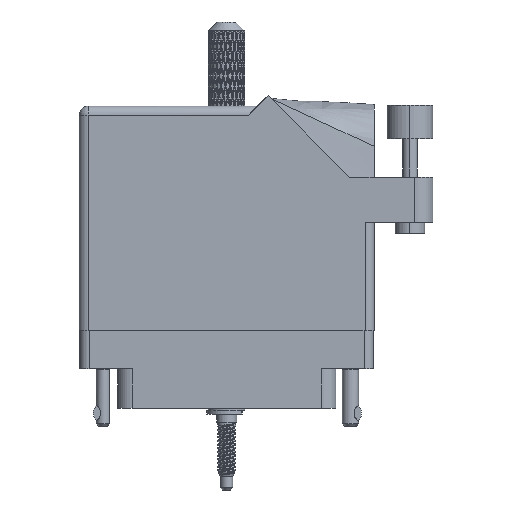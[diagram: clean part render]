
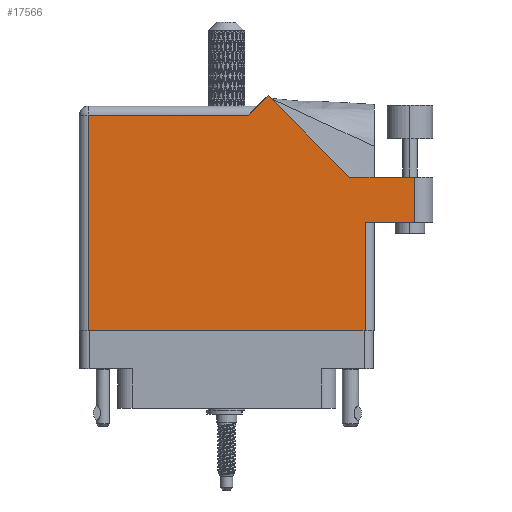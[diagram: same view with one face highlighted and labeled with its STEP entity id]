
A CAD part, front view. The second image highlights one B-rep face of the part: STEP entity #17566.
In plain terms, the highlighted face is planar.
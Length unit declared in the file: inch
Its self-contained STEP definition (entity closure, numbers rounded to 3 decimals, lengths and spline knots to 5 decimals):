
#2791 = DIRECTION ( 'NONE',  ( -0.707, -0.707, 0. ) ) ;
#10307 = LINE ( 'NONE', #37075, #46090 ) ;
#12872 = VERTEX_POINT ( 'NONE', #85176 ) ;
#12920 = DIRECTION ( 'NONE',  ( -1., 0., 0. ) ) ;
#13044 = DIRECTION ( 'NONE',  ( 1., 0., 0. ) ) ;
#15157 = CARTESIAN_POINT ( 'NONE',  ( 1.948, 0.737, 0. ) ) ;
#16138 = AXIS2_PLACEMENT_3D ( 'NONE', #21822, #30300, #65587 ) ;
#16716 = VERTEX_POINT ( 'NONE', #63586 ) ;
#17566 = ADVANCED_FACE ( 'NONE', ( #80615 ), #40283, .F. ) ;
#18502 = DIRECTION ( 'NONE',  ( 0., 1., 0. ) ) ;
#21059 = LINE ( 'NONE', #15157, #89837 ) ;
#21822 = CARTESIAN_POINT ( 'NONE',  ( 0., 1.53, 0. ) ) ;
#22752 = EDGE_LOOP ( 'NONE', ( #46769, #24610, #47847, #94055, #78422, #37450, #82139, #95733, #101850 ) ) ;
#24610 = ORIENTED_EDGE ( 'NONE', *, *, #84553, .T. ) ;
#25171 = EDGE_CURVE ( 'NONE', #108769, #67996, #77918, .T. ) ;
#26047 = CARTESIAN_POINT ( 'NONE',  ( 0., 0., 0. ) ) ;
#26942 = DIRECTION ( 'NONE',  ( -0.707, 0.707, 0. ) ) ;
#28655 = VERTEX_POINT ( 'NONE', #44791 ) ;
#30300 = DIRECTION ( 'NONE',  ( 0., 0., -1. ) ) ;
#32064 = VECTOR ( 'NONE', #40849, 39.37008 ) ;
#32855 = EDGE_CURVE ( 'NONE', #108062, #96433, #21059, .T. ) ;
#32898 = CARTESIAN_POINT ( 'NONE',  ( 1.948, 0., 0. ) ) ;
#34524 = VECTOR ( 'NONE', #43389, 39.37008 ) ;
#34803 = EDGE_CURVE ( 'NONE', #12872, #108062, #49649, .T. ) ;
#35279 = LINE ( 'NONE', #109047, #110829 ) ;
#37075 = CARTESIAN_POINT ( 'NONE',  ( 1.217, 1.53, 0. ) ) ;
#37450 = ORIENTED_EDGE ( 'NONE', *, *, #52442, .T. ) ;
#39596 = CARTESIAN_POINT ( 'NONE',  ( 0.062, 1.468, 0. ) ) ;
#40283 = PLANE ( 'NONE',  #16138 ) ;
#40849 = DIRECTION ( 'NONE',  ( -1., 0., 0. ) ) ;
#41670 = CARTESIAN_POINT ( 'NONE',  ( 0.062, 0., 0. ) ) ;
#43389 = DIRECTION ( 'NONE',  ( 1., 0., 0. ) ) ;
#44791 = CARTESIAN_POINT ( 'NONE',  ( 1.155, 1.468, 0. ) ) ;
#46090 = VECTOR ( 'NONE', #2791, 39.37008 ) ;
#46769 = ORIENTED_EDGE ( 'NONE', *, *, #79324, .T. ) ;
#47406 = CARTESIAN_POINT ( 'NONE',  ( 1.948, 0.737, 0. ) ) ;
#47847 = ORIENTED_EDGE ( 'NONE', *, *, #50066, .T. ) ;
#49649 = LINE ( 'NONE', #26047, #34524 ) ;
#50066 = EDGE_CURVE ( 'NONE', #16716, #108769, #102176, .T. ) ;
#52442 = EDGE_CURVE ( 'NONE', #28655, #72616, #94207, .T. ) ;
#53244 = EDGE_CURVE ( 'NONE', #72616, #12872, #74396, .T. ) ;
#53427 = VERTEX_POINT ( 'NONE', #108708 ) ;
#54209 = CARTESIAN_POINT ( 'NONE',  ( 2.285, 1.044, 0. ) ) ;
#57707 = CARTESIAN_POINT ( 'NONE',  ( 1.28771, 1.60071, 0. ) ) ;
#63586 = CARTESIAN_POINT ( 'NONE',  ( 2.285, 1.044, 0. ) ) ;
#65587 = DIRECTION ( 'NONE',  ( -1., 0., 0. ) ) ;
#67996 = VERTEX_POINT ( 'NONE', #57707 ) ;
#70742 = VECTOR ( 'NONE', #12920, 39.37008 ) ;
#72616 = VERTEX_POINT ( 'NONE', #39596 ) ;
#74396 = LINE ( 'NONE', #41670, #92307 ) ;
#77918 = LINE ( 'NONE', #79149, #104016 ) ;
#78422 = ORIENTED_EDGE ( 'NONE', *, *, #82721, .T. ) ;
#79149 = CARTESIAN_POINT ( 'NONE',  ( 1.84442, 1.044, 0. ) ) ;
#79324 = EDGE_CURVE ( 'NONE', #96433, #53427, #35279, .T. ) ;
#80615 = FACE_OUTER_BOUND ( 'NONE', #22752, .T. ) ;
#82139 = ORIENTED_EDGE ( 'NONE', *, *, #53244, .T. ) ;
#82721 = EDGE_CURVE ( 'NONE', #67996, #28655, #10307, .T. ) ;
#84456 = CARTESIAN_POINT ( 'NONE',  ( 1.84442, 1.044, 0. ) ) ;
#84553 = EDGE_CURVE ( 'NONE', #53427, #16716, #100718, .T. ) ;
#85176 = CARTESIAN_POINT ( 'NONE',  ( 0.062, 0., 0. ) ) ;
#89837 = VECTOR ( 'NONE', #101621, 39.37008 ) ;
#91921 = CARTESIAN_POINT ( 'NONE',  ( 2.41, 1.044, 0. ) ) ;
#92307 = VECTOR ( 'NONE', #110715, 39.37008 ) ;
#94055 = ORIENTED_EDGE ( 'NONE', *, *, #25171, .T. ) ;
#94207 = LINE ( 'NONE', #100516, #70742 ) ;
#95189 = VECTOR ( 'NONE', #18502, 39.37008 ) ;
#95733 = ORIENTED_EDGE ( 'NONE', *, *, #34803, .T. ) ;
#96433 = VERTEX_POINT ( 'NONE', #47406 ) ;
#100516 = CARTESIAN_POINT ( 'NONE',  ( 0., 1.468, 0. ) ) ;
#100718 = LINE ( 'NONE', #54209, #95189 ) ;
#101621 = DIRECTION ( 'NONE',  ( 0., 1., 0. ) ) ;
#101850 = ORIENTED_EDGE ( 'NONE', *, *, #32855, .T. ) ;
#102176 = LINE ( 'NONE', #91921, #32064 ) ;
#104016 = VECTOR ( 'NONE', #26942, 39.37008 ) ;
#108062 = VERTEX_POINT ( 'NONE', #32898 ) ;
#108708 = CARTESIAN_POINT ( 'NONE',  ( 2.285, 0.737, 0. ) ) ;
#108769 = VERTEX_POINT ( 'NONE', #84456 ) ;
#109047 = CARTESIAN_POINT ( 'NONE',  ( 2.01, 0.737, 0. ) ) ;
#110715 = DIRECTION ( 'NONE',  ( 0., -1., 0. ) ) ;
#110829 = VECTOR ( 'NONE', #13044, 39.37008 ) ;
